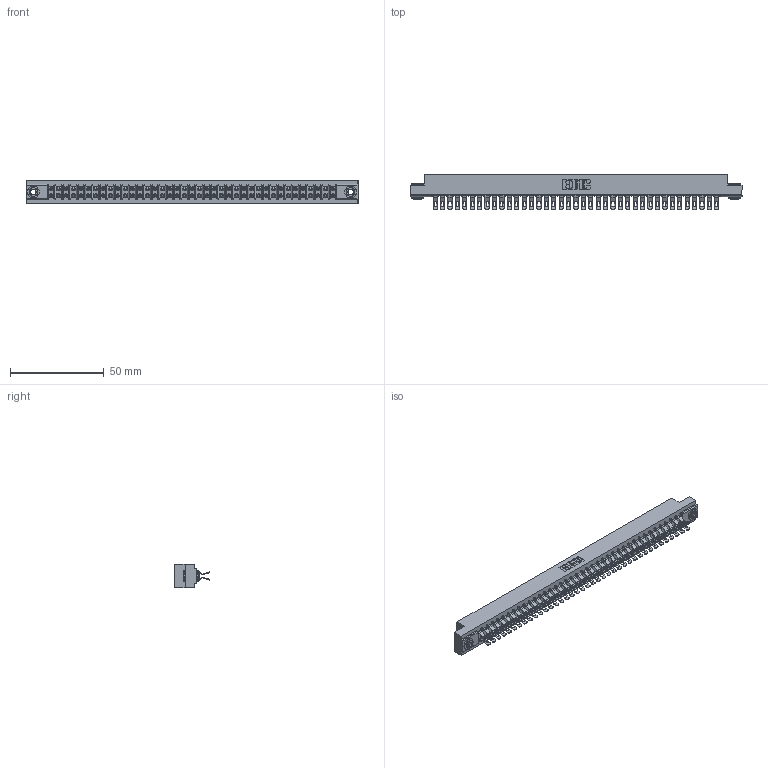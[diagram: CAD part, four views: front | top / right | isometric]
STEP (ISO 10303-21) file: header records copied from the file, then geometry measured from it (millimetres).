
FILE_DESCRIPTION (( 'STEP AP203' ), '1' );
FILE_NAME ('357-078-555-203.STEP', '2019-09-19T14:43:02', ( '' ), ( '' ), 'SwSTEP 2.0', 'SolidWorks 2016', '' );
FILE_SCHEMA (( 'CONFIG_CONTROL_DESIGN' ));
Length unit declared in the file: inch
Products named in the file (4): 307 Part_.156 Dia Mounting Holes; 307-290-001_555; 345-250-002_345-250-002-102; 357-078-555-203
Assembly tree (81 placements, depth 2):
  357-078-555-203
    307 Part_.156 Dia Mounting Holes
    307-290-001_555  x78
    345-250-002_345-250-002-102  x2
Bounding box: 177.55 x 18.75 x 12.7 mm (x, y, z)
Volume: 19092.4 mm3; surface area: 24840.4 mm2
Topology: 81 solids, 81 shells, 4968 faces, 14553 edges, 9486 vertices
Faces by surface type: plane 2746, cylinder 2134, sphere 80, cone 8
Entity records: 36654 total; most frequent: CARTESIAN_POINT 5984, ORIENTED_EDGE 5924, DIRECTION 5884, EDGE_CURVE 2962, VECTOR 2252, LINE 2252, VERTEX_POINT 1916, AXIS2_PLACEMENT_3D 1816
